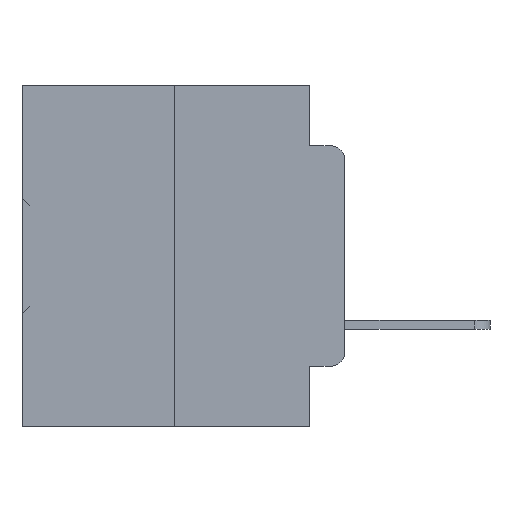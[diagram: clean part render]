
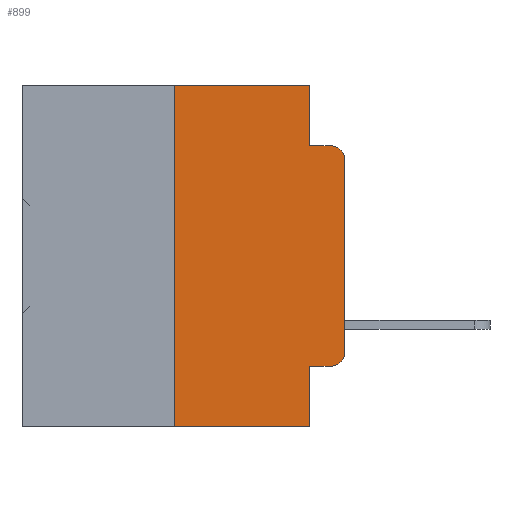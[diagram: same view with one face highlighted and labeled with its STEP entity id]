
A CAD part, left-side view. The second image highlights one B-rep face of the part: STEP entity #899.
In plain terms, the highlighted planar face has unit normal (-1, 0, 0).
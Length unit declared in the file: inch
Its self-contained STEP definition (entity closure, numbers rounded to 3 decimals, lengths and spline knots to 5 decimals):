
#549 = CARTESIAN_POINT ( 'NONE',  ( 0., 0.051, -0.0885 ) ) ;
#758 = CARTESIAN_POINT ( 'NONE',  ( 0., 0.473, 0. ) ) ;
#899 = ADVANCED_FACE ( 'NONE', ( #30702 ), #6610, .F. ) ;
#966 = DIRECTION ( 'NONE',  ( 0., 0., -1. ) ) ;
#1269 = LINE ( 'NONE', #9103, #23577 ) ;
#1414 = VECTOR ( 'NONE', #3865, 39.37008 ) ;
#1682 = EDGE_CURVE ( 'NONE', #10774, #17675, #34121, .T. ) ;
#1933 = CARTESIAN_POINT ( 'NONE',  ( 0., 0.25, -0.5 ) ) ;
#3865 = DIRECTION ( 'NONE',  ( 0., -1., 0. ) ) ;
#3876 = EDGE_CURVE ( 'NONE', #10774, #30473, #1269, .T. ) ;
#4172 = DIRECTION ( 'NONE',  ( 1., 0., 0. ) ) ;
#4208 = DIRECTION ( 'NONE',  ( 0., 0., -1. ) ) ;
#4344 = VECTOR ( 'NONE', #8747, 39.37008 ) ;
#4713 = CARTESIAN_POINT ( 'NONE',  ( 0., 0.473, 0. ) ) ;
#5567 = CARTESIAN_POINT ( 'NONE',  ( 0., 0., 0. ) ) ;
#5917 = CARTESIAN_POINT ( 'NONE',  ( 0., 0.051, 0. ) ) ;
#5985 = CARTESIAN_POINT ( 'NONE',  ( 0., 0.051, -0.0885 ) ) ;
#6491 = EDGE_LOOP ( 'NONE', ( #37039, #16806, #37848, #31380, #33120, #26568, #13147, #14084, #37431, #23580 ) ) ;
#6610 = PLANE ( 'NONE',  #21215 ) ;
#7124 = CARTESIAN_POINT ( 'NONE',  ( 0., 0.02, -0.3915 ) ) ;
#7275 = DIRECTION ( 'NONE',  ( 0., -1., 0. ) ) ;
#7393 = CARTESIAN_POINT ( 'NONE',  ( 0., 0.02, -0.0885 ) ) ;
#7709 = EDGE_CURVE ( 'NONE', #17340, #35143, #31800, .T. ) ;
#7788 = VECTOR ( 'NONE', #7275, 39.37008 ) ;
#8235 = CARTESIAN_POINT ( 'NONE',  ( 0., 0.25, 0. ) ) ;
#8747 = DIRECTION ( 'NONE',  ( 0., 0., 1. ) ) ;
#8761 = CARTESIAN_POINT ( 'NONE',  ( 0., 0., -0.1085 ) ) ;
#8887 = DIRECTION ( 'NONE',  ( 0., 0., -1. ) ) ;
#9103 = CARTESIAN_POINT ( 'NONE',  ( 0., 0.051, 0. ) ) ;
#10264 = DIRECTION ( 'NONE',  ( 0., 0., -1. ) ) ;
#10774 = VERTEX_POINT ( 'NONE', #26699 ) ;
#11177 = CIRCLE ( 'NONE', #36261, 0.02 ) ;
#12660 = LINE ( 'NONE', #5567, #4344 ) ;
#13147 = ORIENTED_EDGE ( 'NONE', *, *, #21680, .T. ) ;
#14084 = ORIENTED_EDGE ( 'NONE', *, *, #3876, .F. ) ;
#15524 = DIRECTION ( 'NONE',  ( 0., -1., 0. ) ) ;
#16249 = VERTEX_POINT ( 'NONE', #1933 ) ;
#16265 = EDGE_CURVE ( 'NONE', #16249, #17340, #34811, .T. ) ;
#16267 = CARTESIAN_POINT ( 'NONE',  ( 0., 0.051, 0. ) ) ;
#16806 = ORIENTED_EDGE ( 'NONE', *, *, #31415, .T. ) ;
#17340 = VERTEX_POINT ( 'NONE', #28943 ) ;
#17675 = VERTEX_POINT ( 'NONE', #24960 ) ;
#18292 = EDGE_CURVE ( 'NONE', #35143, #37444, #19926, .T. ) ;
#19406 = DIRECTION ( 'NONE',  ( 0., 0., -1. ) ) ;
#19506 = DIRECTION ( 'NONE',  ( -1., 0., 0. ) ) ;
#19926 = LINE ( 'NONE', #16267, #26425 ) ;
#20227 = EDGE_CURVE ( 'NONE', #37444, #35872, #25449, .T. ) ;
#21116 = CARTESIAN_POINT ( 'NONE',  ( 0., 0.051, -0.5 ) ) ;
#21215 = AXIS2_PLACEMENT_3D ( 'NONE', #4713, #4172, #4208 ) ;
#21680 = EDGE_CURVE ( 'NONE', #16249, #30473, #34411, .T. ) ;
#22376 = AXIS2_PLACEMENT_3D ( 'NONE', #36171, #19506, #966 ) ;
#23577 = VECTOR ( 'NONE', #8887, 39.37008 ) ;
#23580 = ORIENTED_EDGE ( 'NONE', *, *, #37649, .T. ) ;
#24960 = CARTESIAN_POINT ( 'NONE',  ( 0., 0.02, -0.4115 ) ) ;
#25264 = VERTEX_POINT ( 'NONE', #29119 ) ;
#25449 = LINE ( 'NONE', #549, #1414 ) ;
#26425 = VECTOR ( 'NONE', #19406, 39.37008 ) ;
#26568 = ORIENTED_EDGE ( 'NONE', *, *, #16265, .F. ) ;
#26699 = CARTESIAN_POINT ( 'NONE',  ( 0., 0.051, -0.4115 ) ) ;
#27544 = DIRECTION ( 'NONE',  ( -1., 0., 0. ) ) ;
#27854 = VECTOR ( 'NONE', #15524, 39.37008 ) ;
#28671 = DIRECTION ( 'NONE',  ( 0., 0., 1. ) ) ;
#28943 = CARTESIAN_POINT ( 'NONE',  ( 0., 0.25, 0. ) ) ;
#29119 = CARTESIAN_POINT ( 'NONE',  ( 0., 0., -0.3915 ) ) ;
#29600 = CARTESIAN_POINT ( 'NONE',  ( 0., 0.473, -0.5 ) ) ;
#30473 = VERTEX_POINT ( 'NONE', #21116 ) ;
#30702 = FACE_OUTER_BOUND ( 'NONE', #6491, .T. ) ;
#31380 = ORIENTED_EDGE ( 'NONE', *, *, #18292, .F. ) ;
#31415 = EDGE_CURVE ( 'NONE', #37364, #35872, #35016, .T. ) ;
#31800 = LINE ( 'NONE', #758, #7788 ) ;
#33120 = ORIENTED_EDGE ( 'NONE', *, *, #7709, .F. ) ;
#33256 = VECTOR ( 'NONE', #36197, 39.37008 ) ;
#33283 = EDGE_CURVE ( 'NONE', #25264, #37364, #12660, .T. ) ;
#33939 = VECTOR ( 'NONE', #28671, 39.37008 ) ;
#34121 = LINE ( 'NONE', #36274, #33256 ) ;
#34411 = LINE ( 'NONE', #29600, #27854 ) ;
#34811 = LINE ( 'NONE', #8235, #33939 ) ;
#35016 = CIRCLE ( 'NONE', #22376, 0.02 ) ;
#35143 = VERTEX_POINT ( 'NONE', #5917 ) ;
#35872 = VERTEX_POINT ( 'NONE', #7393 ) ;
#36171 = CARTESIAN_POINT ( 'NONE',  ( 0., 0.02, -0.1085 ) ) ;
#36197 = DIRECTION ( 'NONE',  ( 0., -1., 0. ) ) ;
#36261 = AXIS2_PLACEMENT_3D ( 'NONE', #7124, #27544, #10264 ) ;
#36274 = CARTESIAN_POINT ( 'NONE',  ( 0., 0.051, -0.4115 ) ) ;
#37039 = ORIENTED_EDGE ( 'NONE', *, *, #33283, .T. ) ;
#37364 = VERTEX_POINT ( 'NONE', #8761 ) ;
#37431 = ORIENTED_EDGE ( 'NONE', *, *, #1682, .T. ) ;
#37444 = VERTEX_POINT ( 'NONE', #5985 ) ;
#37649 = EDGE_CURVE ( 'NONE', #17675, #25264, #11177, .T. ) ;
#37848 = ORIENTED_EDGE ( 'NONE', *, *, #20227, .F. ) ;
